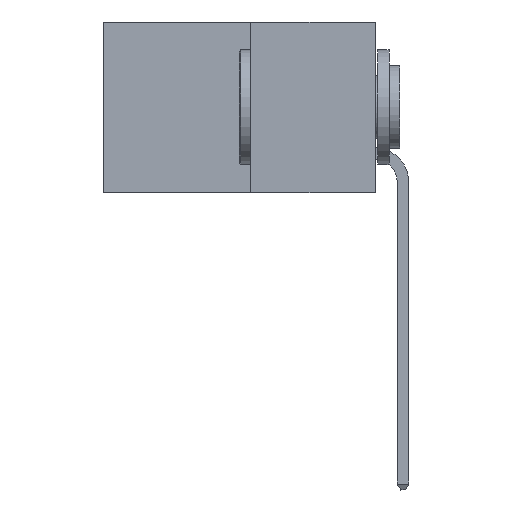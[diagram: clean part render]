
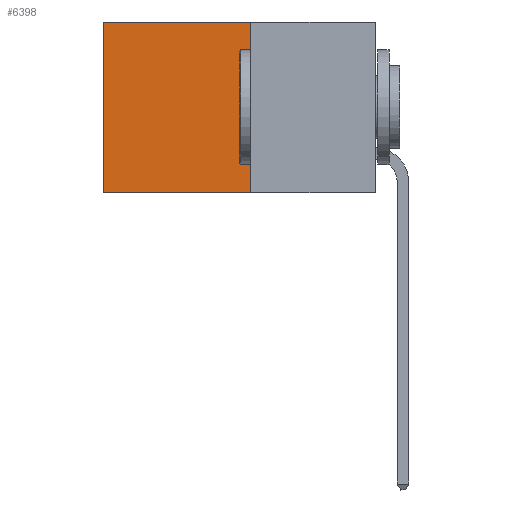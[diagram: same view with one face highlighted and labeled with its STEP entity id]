
A CAD part, left-side view. The second image highlights one B-rep face of the part: STEP entity #6398.
In plain terms, the highlighted planar face has unit normal (-1, 0, 0).
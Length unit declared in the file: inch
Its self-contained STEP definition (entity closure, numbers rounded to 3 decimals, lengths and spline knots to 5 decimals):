
#558 = VERTEX_POINT ( 'NONE', #994 ) ;
#994 = CARTESIAN_POINT ( 'NONE',  ( 0.277, 0.27, -0.37 ) ) ;
#1126 = EDGE_CURVE ( 'NONE', #6942, #558, #7978, .T. ) ;
#1422 = ORIENTED_EDGE ( 'NONE', *, *, #4240, .T. ) ;
#2130 = LINE ( 'NONE', #6452, #17879 ) ;
#2418 = VECTOR ( 'NONE', #6949, 39.37008 ) ;
#3453 = ORIENTED_EDGE ( 'NONE', *, *, #1126, .F. ) ;
#3773 = CARTESIAN_POINT ( 'NONE',  ( 0.277, 0.27, 0. ) ) ;
#4240 = EDGE_CURVE ( 'NONE', #17926, #4620, #20229, .T. ) ;
#4620 = VERTEX_POINT ( 'NONE', #12233 ) ;
#6398 = ADVANCED_FACE ( 'NONE', ( #15229 ), #11427, .F. ) ;
#6452 = CARTESIAN_POINT ( 'NONE',  ( 0.277, 0.27, -0.37 ) ) ;
#6942 = VERTEX_POINT ( 'NONE', #3773 ) ;
#6949 = DIRECTION ( 'NONE',  ( 0., 0., -1. ) ) ;
#7978 = LINE ( 'NONE', #10061, #2418 ) ;
#8507 = DIRECTION ( 'NONE',  ( 0., 1., 0. ) ) ;
#9997 = CARTESIAN_POINT ( 'NONE',  ( 0.277, 0.27, 0. ) ) ;
#10061 = CARTESIAN_POINT ( 'NONE',  ( 0.277, 0.27, -0.37 ) ) ;
#11400 = DIRECTION ( 'NONE',  ( 1., 0., 0. ) ) ;
#11427 = PLANE ( 'NONE',  #13338 ) ;
#11673 = CARTESIAN_POINT ( 'NONE',  ( 0.277, 0.59, 0. ) ) ;
#12066 = DIRECTION ( 'NONE',  ( 0., 1., 0. ) ) ;
#12075 = CARTESIAN_POINT ( 'NONE',  ( 0.277, 0.27, -0.37 ) ) ;
#12233 = CARTESIAN_POINT ( 'NONE',  ( 0.277, 0.59, -0.37 ) ) ;
#12320 = DIRECTION ( 'NONE',  ( 0., 0., -1. ) ) ;
#12643 = LINE ( 'NONE', #9997, #22683 ) ;
#13338 = AXIS2_PLACEMENT_3D ( 'NONE', #12075, #11400, #12320 ) ;
#14108 = EDGE_LOOP ( 'NONE', ( #1422, #18332, #3453, #16660 ) ) ;
#14895 = VECTOR ( 'NONE', #23502, 39.37008 ) ;
#15229 = FACE_OUTER_BOUND ( 'NONE', #14108, .T. ) ;
#15658 = EDGE_CURVE ( 'NONE', #558, #4620, #2130, .T. ) ;
#16660 = ORIENTED_EDGE ( 'NONE', *, *, #21343, .T. ) ;
#17879 = VECTOR ( 'NONE', #8507, 39.37008 ) ;
#17926 = VERTEX_POINT ( 'NONE', #11673 ) ;
#18332 = ORIENTED_EDGE ( 'NONE', *, *, #15658, .F. ) ;
#20229 = LINE ( 'NONE', #24162, #14895 ) ;
#21343 = EDGE_CURVE ( 'NONE', #6942, #17926, #12643, .T. ) ;
#22683 = VECTOR ( 'NONE', #12066, 39.37008 ) ;
#23502 = DIRECTION ( 'NONE',  ( 0., 0., -1. ) ) ;
#24162 = CARTESIAN_POINT ( 'NONE',  ( 0.277, 0.59, -0.37 ) ) ;
